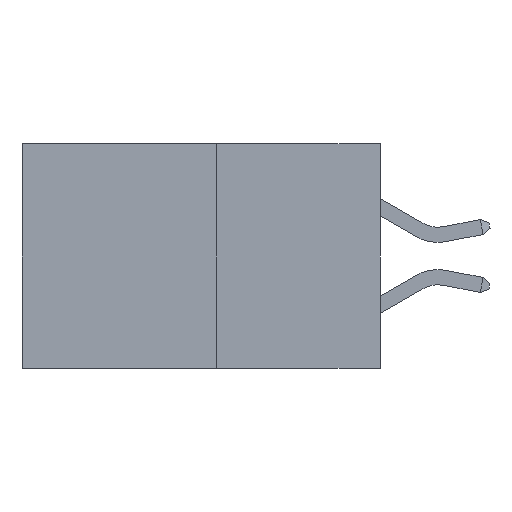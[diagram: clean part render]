
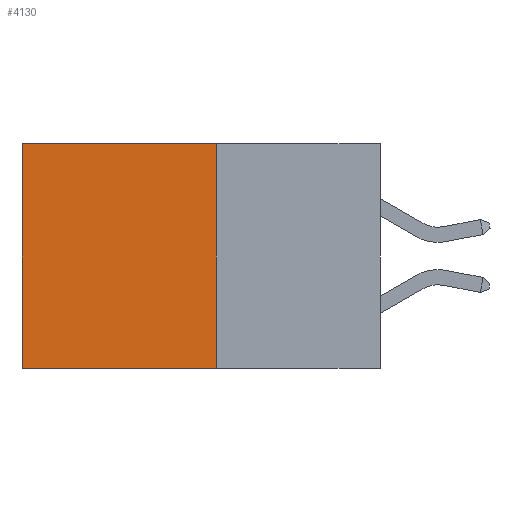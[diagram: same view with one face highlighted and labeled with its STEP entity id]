
A CAD part, left-side view. The second image highlights one B-rep face of the part: STEP entity #4130.
In plain terms, the highlighted planar face has unit normal (-1, 0, 0).
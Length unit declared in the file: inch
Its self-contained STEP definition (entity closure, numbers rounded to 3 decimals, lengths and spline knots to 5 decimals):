
#113 = VECTOR ( 'NONE', #23169, 39.37008 ) ;
#1508 = EDGE_CURVE ( 'NONE', #15801, #2226, #3522, .T. ) ;
#1874 = ORIENTED_EDGE ( 'NONE', *, *, #1508, .T. ) ;
#2226 = VERTEX_POINT ( 'NONE', #2564 ) ;
#2564 = CARTESIAN_POINT ( 'NONE',  ( 0.277, 0.59, 0. ) ) ;
#2796 = VECTOR ( 'NONE', #26454, 39.37008 ) ;
#3522 = LINE ( 'NONE', #19360, #2796 ) ;
#4130 = ADVANCED_FACE ( 'NONE', ( #15065 ), #5571, .F. ) ;
#5181 = DIRECTION ( 'NONE',  ( 0., 0., -1. ) ) ;
#5412 = DIRECTION ( 'NONE',  ( 1., 0., 0. ) ) ;
#5571 = PLANE ( 'NONE',  #27113 ) ;
#5579 = DIRECTION ( 'NONE',  ( 0., 0., -1. ) ) ;
#5581 = LINE ( 'NONE', #10293, #113 ) ;
#5791 = CARTESIAN_POINT ( 'NONE',  ( 0.277, 0.27, -0.37 ) ) ;
#6373 = ORIENTED_EDGE ( 'NONE', *, *, #12886, .F. ) ;
#7068 = LINE ( 'NONE', #16446, #12199 ) ;
#7986 = CARTESIAN_POINT ( 'NONE',  ( 0.277, 0.27, -0.37 ) ) ;
#10293 = CARTESIAN_POINT ( 'NONE',  ( 0.277, 0.27, -0.37 ) ) ;
#10381 = EDGE_CURVE ( 'NONE', #2226, #23354, #7068, .T. ) ;
#10440 = LINE ( 'NONE', #7986, #16187 ) ;
#11300 = EDGE_CURVE ( 'NONE', #15801, #23232, #10440, .T. ) ;
#12199 = VECTOR ( 'NONE', #5579, 39.37008 ) ;
#12886 = EDGE_CURVE ( 'NONE', #23232, #23354, #5581, .T. ) ;
#14937 = CARTESIAN_POINT ( 'NONE',  ( 0.277, 0.59, -0.37 ) ) ;
#15065 = FACE_OUTER_BOUND ( 'NONE', #27916, .T. ) ;
#15801 = VERTEX_POINT ( 'NONE', #16400 ) ;
#16187 = VECTOR ( 'NONE', #27324, 39.37008 ) ;
#16400 = CARTESIAN_POINT ( 'NONE',  ( 0.277, 0.27, 0. ) ) ;
#16446 = CARTESIAN_POINT ( 'NONE',  ( 0.277, 0.59, -0.37 ) ) ;
#19360 = CARTESIAN_POINT ( 'NONE',  ( 0.277, 0.27, 0. ) ) ;
#21498 = ORIENTED_EDGE ( 'NONE', *, *, #11300, .F. ) ;
#23169 = DIRECTION ( 'NONE',  ( 0., 1., 0. ) ) ;
#23232 = VERTEX_POINT ( 'NONE', #25309 ) ;
#23354 = VERTEX_POINT ( 'NONE', #14937 ) ;
#25309 = CARTESIAN_POINT ( 'NONE',  ( 0.277, 0.27, -0.37 ) ) ;
#26454 = DIRECTION ( 'NONE',  ( 0., 1., 0. ) ) ;
#26599 = ORIENTED_EDGE ( 'NONE', *, *, #10381, .T. ) ;
#27113 = AXIS2_PLACEMENT_3D ( 'NONE', #5791, #5412, #5181 ) ;
#27324 = DIRECTION ( 'NONE',  ( 0., 0., -1. ) ) ;
#27916 = EDGE_LOOP ( 'NONE', ( #26599, #6373, #21498, #1874 ) ) ;
